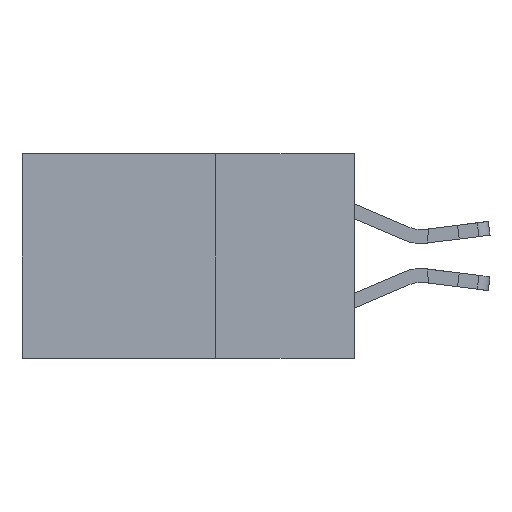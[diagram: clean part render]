
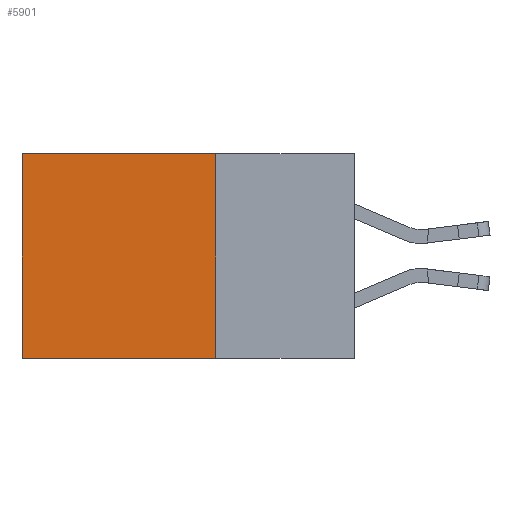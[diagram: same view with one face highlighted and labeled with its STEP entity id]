
A CAD part, left-side view. The second image highlights one B-rep face of the part: STEP entity #5901.
In plain terms, the highlighted planar face has unit normal (-1, 0, 0).
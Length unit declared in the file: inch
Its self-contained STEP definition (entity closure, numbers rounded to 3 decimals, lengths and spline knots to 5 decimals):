
#96 = CARTESIAN_POINT ( 'NONE',  ( 0.2615, 0.25, -0.37 ) ) ;
#124 = VERTEX_POINT ( 'NONE', #8787 ) ;
#262 = LINE ( 'NONE', #7224, #3272 ) ;
#1190 = LINE ( 'NONE', #11655, #12942 ) ;
#1441 = VECTOR ( 'NONE', #5081, 39.37008 ) ;
#1711 = EDGE_LOOP ( 'NONE', ( #2307, #2519, #12081, #7886 ) ) ;
#2307 = ORIENTED_EDGE ( 'NONE', *, *, #8836, .T. ) ;
#2484 = VECTOR ( 'NONE', #14273, 39.37008 ) ;
#2519 = ORIENTED_EDGE ( 'NONE', *, *, #5933, .F. ) ;
#3209 = VERTEX_POINT ( 'NONE', #8293 ) ;
#3272 = VECTOR ( 'NONE', #12193, 39.37008 ) ;
#3502 = VERTEX_POINT ( 'NONE', #15328 ) ;
#3858 = PLANE ( 'NONE',  #10795 ) ;
#4790 = CARTESIAN_POINT ( 'NONE',  ( 0.2615, 0.25, -0.37 ) ) ;
#5081 = DIRECTION ( 'NONE',  ( 0., 1., 0. ) ) ;
#5494 = DIRECTION ( 'NONE',  ( 0., 1., 0. ) ) ;
#5901 = ADVANCED_FACE ( 'NONE', ( #7427 ), #3858, .F. ) ;
#5933 = EDGE_CURVE ( 'NONE', #3502, #15828, #15991, .T. ) ;
#7224 = CARTESIAN_POINT ( 'NONE',  ( 0.2615, 0.25, -0.37 ) ) ;
#7427 = FACE_OUTER_BOUND ( 'NONE', #1711, .T. ) ;
#7502 = EDGE_CURVE ( 'NONE', #3209, #124, #1190, .T. ) ;
#7886 = ORIENTED_EDGE ( 'NONE', *, *, #7502, .T. ) ;
#7967 = CARTESIAN_POINT ( 'NONE',  ( 0.2615, 0.6, -0.37 ) ) ;
#8293 = CARTESIAN_POINT ( 'NONE',  ( 0.2615, 0.25, 0. ) ) ;
#8738 = EDGE_CURVE ( 'NONE', #3209, #3502, #262, .T. ) ;
#8787 = CARTESIAN_POINT ( 'NONE',  ( 0.2615, 0.6, 0. ) ) ;
#8836 = EDGE_CURVE ( 'NONE', #124, #15828, #10447, .T. ) ;
#9728 = DIRECTION ( 'NONE',  ( 0., 0., -1. ) ) ;
#10447 = LINE ( 'NONE', #10600, #2484 ) ;
#10600 = CARTESIAN_POINT ( 'NONE',  ( 0.2615, 0.6, -0.37 ) ) ;
#10795 = AXIS2_PLACEMENT_3D ( 'NONE', #4790, #12405, #9728 ) ;
#11655 = CARTESIAN_POINT ( 'NONE',  ( 0.2615, 0.25, 0. ) ) ;
#12081 = ORIENTED_EDGE ( 'NONE', *, *, #8738, .F. ) ;
#12193 = DIRECTION ( 'NONE',  ( 0., 0., -1. ) ) ;
#12405 = DIRECTION ( 'NONE',  ( 1., 0., 0. ) ) ;
#12942 = VECTOR ( 'NONE', #5494, 39.37008 ) ;
#14273 = DIRECTION ( 'NONE',  ( 0., 0., -1. ) ) ;
#15328 = CARTESIAN_POINT ( 'NONE',  ( 0.2615, 0.25, -0.37 ) ) ;
#15828 = VERTEX_POINT ( 'NONE', #7967 ) ;
#15991 = LINE ( 'NONE', #96, #1441 ) ;
